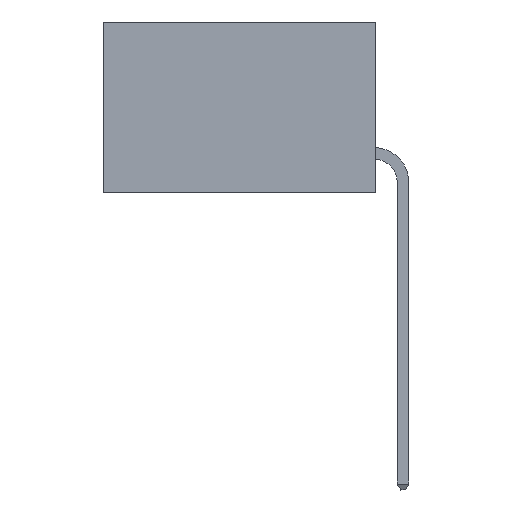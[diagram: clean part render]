
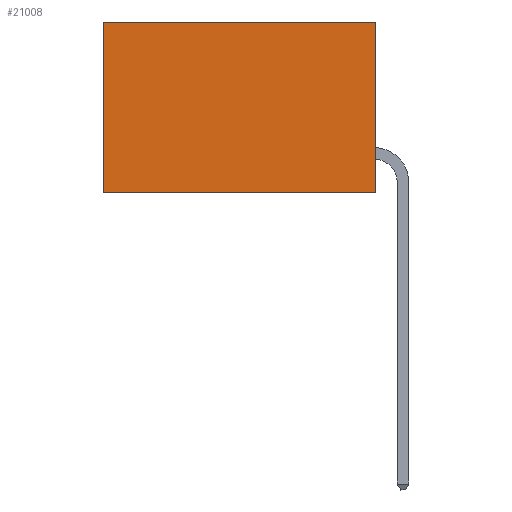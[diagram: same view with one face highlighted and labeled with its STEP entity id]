
A CAD part, left-side view. The second image highlights one B-rep face of the part: STEP entity #21008.
In plain terms, the highlighted planar face has unit normal (-1, 0, 0).
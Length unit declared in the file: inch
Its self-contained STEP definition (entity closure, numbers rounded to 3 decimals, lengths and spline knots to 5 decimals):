
#904 = ORIENTED_EDGE ( 'NONE', *, *, #8854, .T. ) ;
#1234 = CARTESIAN_POINT ( 'NONE',  ( 0.277, 0., -0.37 ) ) ;
#3132 = PLANE ( 'NONE',  #29401 ) ;
#3212 = LINE ( 'NONE', #29335, #21421 ) ;
#3704 = DIRECTION ( 'NONE',  ( 0., 1., 0. ) ) ;
#5413 = VECTOR ( 'NONE', #3704, 39.37008 ) ;
#6420 = DIRECTION ( 'NONE',  ( 0., 0., -1. ) ) ;
#8129 = DIRECTION ( 'NONE',  ( 0., 0., -1. ) ) ;
#8854 = EDGE_CURVE ( 'NONE', #15644, #23680, #29426, .T. ) ;
#9353 = ORIENTED_EDGE ( 'NONE', *, *, #25072, .F. ) ;
#9613 = VECTOR ( 'NONE', #30676, 39.37008 ) ;
#9810 = VECTOR ( 'NONE', #6420, 39.37008 ) ;
#11037 = FACE_OUTER_BOUND ( 'NONE', #17073, .T. ) ;
#11667 = CARTESIAN_POINT ( 'NONE',  ( 0.277, 0., -0.37 ) ) ;
#12573 = EDGE_CURVE ( 'NONE', #23680, #13211, #3212, .T. ) ;
#13211 = VERTEX_POINT ( 'NONE', #27193 ) ;
#15644 = VERTEX_POINT ( 'NONE', #32039 ) ;
#16369 = LINE ( 'NONE', #18748, #9810 ) ;
#17073 = EDGE_LOOP ( 'NONE', ( #30531, #29555, #9353, #904 ) ) ;
#17355 = EDGE_CURVE ( 'NONE', #32027, #13211, #25160, .T. ) ;
#18748 = CARTESIAN_POINT ( 'NONE',  ( 0.277, 0., -0.37 ) ) ;
#20475 = CARTESIAN_POINT ( 'NONE',  ( 0.277, 0., -0.37 ) ) ;
#21008 = ADVANCED_FACE ( 'NONE', ( #11037 ), #3132, .F. ) ;
#21421 = VECTOR ( 'NONE', #26777, 39.37008 ) ;
#22931 = DIRECTION ( 'NONE',  ( 1., 0., 0. ) ) ;
#23680 = VERTEX_POINT ( 'NONE', #28715 ) ;
#25072 = EDGE_CURVE ( 'NONE', #15644, #32027, #16369, .T. ) ;
#25160 = LINE ( 'NONE', #1234, #5413 ) ;
#26777 = DIRECTION ( 'NONE',  ( 0., 0., -1. ) ) ;
#27193 = CARTESIAN_POINT ( 'NONE',  ( 0.277, 0.59, -0.37 ) ) ;
#28715 = CARTESIAN_POINT ( 'NONE',  ( 0.277, 0.59, 0. ) ) ;
#29335 = CARTESIAN_POINT ( 'NONE',  ( 0.277, 0.59, -0.37 ) ) ;
#29401 = AXIS2_PLACEMENT_3D ( 'NONE', #20475, #22931, #8129 ) ;
#29426 = LINE ( 'NONE', #31302, #9613 ) ;
#29555 = ORIENTED_EDGE ( 'NONE', *, *, #17355, .F. ) ;
#30531 = ORIENTED_EDGE ( 'NONE', *, *, #12573, .T. ) ;
#30676 = DIRECTION ( 'NONE',  ( 0., 1., 0. ) ) ;
#31302 = CARTESIAN_POINT ( 'NONE',  ( 0.277, 0., 0. ) ) ;
#32027 = VERTEX_POINT ( 'NONE', #11667 ) ;
#32039 = CARTESIAN_POINT ( 'NONE',  ( 0.277, 0., 0. ) ) ;
